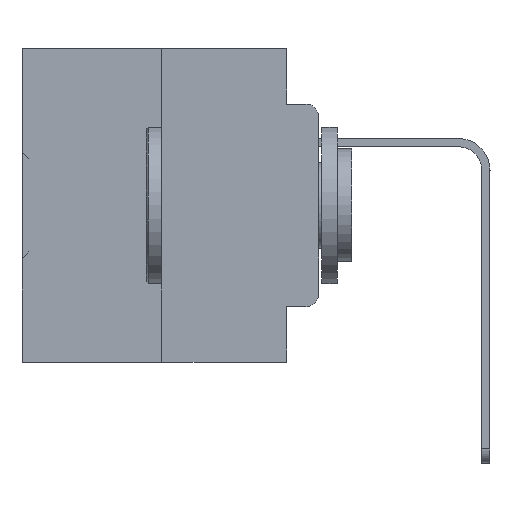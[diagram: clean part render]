
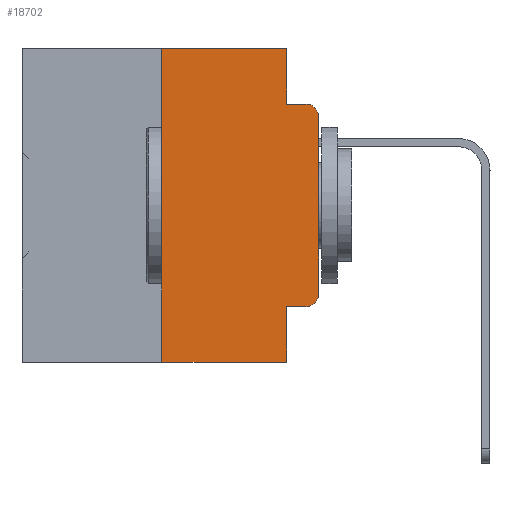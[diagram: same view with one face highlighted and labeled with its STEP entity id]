
A CAD part, left-side view. The second image highlights one B-rep face of the part: STEP entity #18702.
In plain terms, the highlighted planar face has unit normal (-1, 0, 0).
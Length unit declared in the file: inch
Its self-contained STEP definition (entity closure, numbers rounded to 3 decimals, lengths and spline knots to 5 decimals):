
#176 = VERTEX_POINT ( 'NONE', #23327 ) ;
#282 = DIRECTION ( 'NONE',  ( 0., 0., -1. ) ) ;
#324 = CARTESIAN_POINT ( 'NONE',  ( 0., 0.25, 0. ) ) ;
#968 = ORIENTED_EDGE ( 'NONE', *, *, #27560, .F. ) ;
#1150 = VERTEX_POINT ( 'NONE', #15574 ) ;
#1207 = EDGE_CURVE ( 'NONE', #10763, #176, #30171, .T. ) ;
#1244 = CARTESIAN_POINT ( 'NONE',  ( 0., 0., -0.1085 ) ) ;
#1536 = AXIS2_PLACEMENT_3D ( 'NONE', #8965, #9229, #282 ) ;
#2150 = DIRECTION ( 'NONE',  ( 0., -1., 0. ) ) ;
#2293 = CARTESIAN_POINT ( 'NONE',  ( 0., 0.473, 0. ) ) ;
#4070 = LINE ( 'NONE', #9309, #28819 ) ;
#5226 = DIRECTION ( 'NONE',  ( 0., -1., 0. ) ) ;
#5335 = LINE ( 'NONE', #30909, #35990 ) ;
#6986 = ORIENTED_EDGE ( 'NONE', *, *, #33000, .T. ) ;
#7589 = VERTEX_POINT ( 'NONE', #28697 ) ;
#7761 = CARTESIAN_POINT ( 'NONE',  ( 0., 0.02, -0.4115 ) ) ;
#7893 = VERTEX_POINT ( 'NONE', #1244 ) ;
#8037 = ORIENTED_EDGE ( 'NONE', *, *, #28352, .T. ) ;
#8841 = EDGE_CURVE ( 'NONE', #35450, #176, #35685, .T. ) ;
#8965 = CARTESIAN_POINT ( 'NONE',  ( 0., 0.02, -0.1085 ) ) ;
#9229 = DIRECTION ( 'NONE',  ( -1., 0., 0. ) ) ;
#9309 = CARTESIAN_POINT ( 'NONE',  ( 0., 0.051, -0.4115 ) ) ;
#9609 = VERTEX_POINT ( 'NONE', #28429 ) ;
#9800 = ORIENTED_EDGE ( 'NONE', *, *, #16586, .T. ) ;
#10763 = VERTEX_POINT ( 'NONE', #27587 ) ;
#10883 = DIRECTION ( 'NONE',  ( 0., 0., -1. ) ) ;
#11432 = VECTOR ( 'NONE', #30269, 39.37008 ) ;
#11478 = VERTEX_POINT ( 'NONE', #25610 ) ;
#12474 = ORIENTED_EDGE ( 'NONE', *, *, #36932, .T. ) ;
#12748 = DIRECTION ( 'NONE',  ( 0., 0., 1. ) ) ;
#13567 = CARTESIAN_POINT ( 'NONE',  ( 0., 0.051, 0. ) ) ;
#14153 = LINE ( 'NONE', #2293, #36990 ) ;
#14184 = LINE ( 'NONE', #25960, #16014 ) ;
#14515 = ORIENTED_EDGE ( 'NONE', *, *, #34748, .F. ) ;
#15574 = CARTESIAN_POINT ( 'NONE',  ( 0., 0.051, -0.0885 ) ) ;
#15641 = ORIENTED_EDGE ( 'NONE', *, *, #1207, .T. ) ;
#16014 = VECTOR ( 'NONE', #2150, 39.37008 ) ;
#16586 = EDGE_CURVE ( 'NONE', #7893, #9609, #26504, .T. ) ;
#16778 = AXIS2_PLACEMENT_3D ( 'NONE', #25824, #17115, #34227 ) ;
#16947 = ORIENTED_EDGE ( 'NONE', *, *, #36771, .F. ) ;
#17115 = DIRECTION ( 'NONE',  ( 1., 0., 0. ) ) ;
#17458 = VERTEX_POINT ( 'NONE', #7761 ) ;
#18702 = ADVANCED_FACE ( 'NONE', ( #36799 ), #25696, .F. ) ;
#19725 = LINE ( 'NONE', #324, #30676 ) ;
#20237 = DIRECTION ( 'NONE',  ( 0., 0., -1. ) ) ;
#21082 = VECTOR ( 'NONE', #20237, 39.37008 ) ;
#21828 = EDGE_CURVE ( 'NONE', #1150, #9609, #14184, .T. ) ;
#22521 = CARTESIAN_POINT ( 'NONE',  ( 0., 0.051, 0. ) ) ;
#23327 = CARTESIAN_POINT ( 'NONE',  ( 0., 0.051, -0.5 ) ) ;
#23375 = EDGE_LOOP ( 'NONE', ( #12474, #9800, #26865, #16947, #14515, #968, #15641, #28159, #8037, #6986 ) ) ;
#24067 = LINE ( 'NONE', #26191, #27755 ) ;
#25078 = DIRECTION ( 'NONE',  ( -1., 0., 0. ) ) ;
#25125 = VERTEX_POINT ( 'NONE', #13567 ) ;
#25592 = CARTESIAN_POINT ( 'NONE',  ( 0., 0.02, -0.3915 ) ) ;
#25610 = CARTESIAN_POINT ( 'NONE',  ( 0., 0.25, 0. ) ) ;
#25696 = PLANE ( 'NONE',  #16778 ) ;
#25824 = CARTESIAN_POINT ( 'NONE',  ( 0., 0.473, 0. ) ) ;
#25960 = CARTESIAN_POINT ( 'NONE',  ( 0., 0.051, -0.0885 ) ) ;
#26014 = AXIS2_PLACEMENT_3D ( 'NONE', #25592, #25078, #10883 ) ;
#26191 = CARTESIAN_POINT ( 'NONE',  ( 0., 0., 0. ) ) ;
#26504 = CIRCLE ( 'NONE', #1536, 0.02 ) ;
#26865 = ORIENTED_EDGE ( 'NONE', *, *, #21828, .F. ) ;
#27560 = EDGE_CURVE ( 'NONE', #10763, #11478, #19725, .T. ) ;
#27587 = CARTESIAN_POINT ( 'NONE',  ( 0., 0.25, -0.5 ) ) ;
#27755 = VECTOR ( 'NONE', #37418, 39.37008 ) ;
#28159 = ORIENTED_EDGE ( 'NONE', *, *, #8841, .F. ) ;
#28352 = EDGE_CURVE ( 'NONE', #35450, #17458, #4070, .T. ) ;
#28429 = CARTESIAN_POINT ( 'NONE',  ( 0., 0.02, -0.0885 ) ) ;
#28697 = CARTESIAN_POINT ( 'NONE',  ( 0., 0., -0.3915 ) ) ;
#28819 = VECTOR ( 'NONE', #32835, 39.37008 ) ;
#29787 = CARTESIAN_POINT ( 'NONE',  ( 0., 0.473, -0.5 ) ) ;
#30171 = LINE ( 'NONE', #29787, #11432 ) ;
#30269 = DIRECTION ( 'NONE',  ( 0., -1., 0. ) ) ;
#30676 = VECTOR ( 'NONE', #12748, 39.37008 ) ;
#30909 = CARTESIAN_POINT ( 'NONE',  ( 0., 0.051, 0. ) ) ;
#31168 = DIRECTION ( 'NONE',  ( 0., 0., -1. ) ) ;
#32835 = DIRECTION ( 'NONE',  ( 0., -1., 0. ) ) ;
#33000 = EDGE_CURVE ( 'NONE', #17458, #7589, #34004, .T. ) ;
#34004 = CIRCLE ( 'NONE', #26014, 0.02 ) ;
#34227 = DIRECTION ( 'NONE',  ( 0., 0., -1. ) ) ;
#34455 = CARTESIAN_POINT ( 'NONE',  ( 0., 0.051, -0.4115 ) ) ;
#34748 = EDGE_CURVE ( 'NONE', #11478, #25125, #14153, .T. ) ;
#35450 = VERTEX_POINT ( 'NONE', #34455 ) ;
#35685 = LINE ( 'NONE', #22521, #21082 ) ;
#35990 = VECTOR ( 'NONE', #31168, 39.37008 ) ;
#36771 = EDGE_CURVE ( 'NONE', #25125, #1150, #5335, .T. ) ;
#36799 = FACE_OUTER_BOUND ( 'NONE', #23375, .T. ) ;
#36932 = EDGE_CURVE ( 'NONE', #7589, #7893, #24067, .T. ) ;
#36990 = VECTOR ( 'NONE', #5226, 39.37008 ) ;
#37418 = DIRECTION ( 'NONE',  ( 0., 0., 1. ) ) ;
